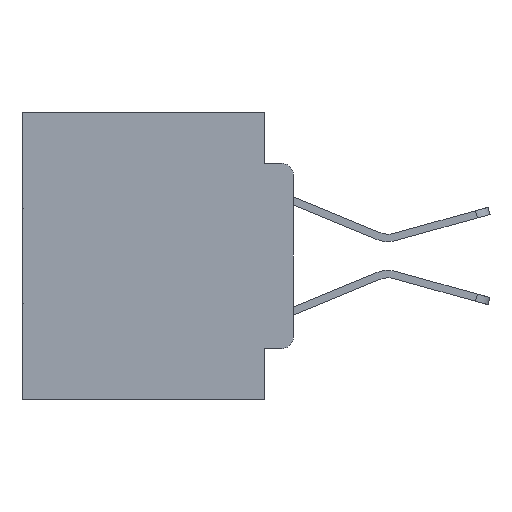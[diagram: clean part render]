
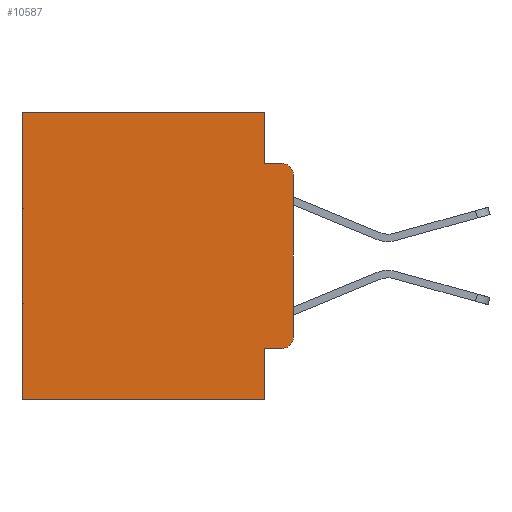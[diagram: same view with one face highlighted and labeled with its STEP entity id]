
A CAD part, left-side view. The second image highlights one B-rep face of the part: STEP entity #10587.
In plain terms, the highlighted planar face has unit normal (-1, 0, 0).
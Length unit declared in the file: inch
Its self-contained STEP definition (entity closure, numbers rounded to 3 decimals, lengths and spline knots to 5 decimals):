
#143 = CARTESIAN_POINT ( 'NONE',  ( 0.298, 0.02, -0.0885 ) ) ;
#873 = DIRECTION ( 'NONE',  ( 0., -1., 0. ) ) ;
#1125 = CARTESIAN_POINT ( 'NONE',  ( 0.298, 0.051, -0.0885 ) ) ;
#1357 = VERTEX_POINT ( 'NONE', #6436 ) ;
#2294 = DIRECTION ( 'NONE',  ( -1., 0., 0. ) ) ;
#2396 = CARTESIAN_POINT ( 'NONE',  ( 0.298, 0.051, -0.4115 ) ) ;
#3027 = AXIS2_PLACEMENT_3D ( 'NONE', #17320, #2294, #19782 ) ;
#3093 = ORIENTED_EDGE ( 'NONE', *, *, #9469, .F. ) ;
#3210 = EDGE_CURVE ( 'NONE', #11670, #21237, #19409, .T. ) ;
#3668 = CARTESIAN_POINT ( 'NONE',  ( 0.298, 0.051, 0. ) ) ;
#4072 = DIRECTION ( 'NONE',  ( -1., 0., 0. ) ) ;
#4357 = CARTESIAN_POINT ( 'NONE',  ( 0.298, 0., 0. ) ) ;
#4598 = ORIENTED_EDGE ( 'NONE', *, *, #27001, .F. ) ;
#5190 = VECTOR ( 'NONE', #873, 39.37008 ) ;
#5524 = EDGE_CURVE ( 'NONE', #11444, #10542, #6011, .T. ) ;
#6011 = LINE ( 'NONE', #9923, #5190 ) ;
#6436 = CARTESIAN_POINT ( 'NONE',  ( 0.298, 0.051, 0. ) ) ;
#6443 = CARTESIAN_POINT ( 'NONE',  ( 0.298, 0.051, -0.4115 ) ) ;
#6484 = VECTOR ( 'NONE', #22529, 39.37008 ) ;
#7074 = VERTEX_POINT ( 'NONE', #31176 ) ;
#7345 = CARTESIAN_POINT ( 'NONE',  ( 0.298, 0.051, 0. ) ) ;
#9018 = AXIS2_PLACEMENT_3D ( 'NONE', #19040, #4072, #21512 ) ;
#9428 = ORIENTED_EDGE ( 'NONE', *, *, #3210, .T. ) ;
#9469 = EDGE_CURVE ( 'NONE', #10667, #11246, #15210, .T. ) ;
#9923 = CARTESIAN_POINT ( 'NONE',  ( 0.298, 0.051, -0.0885 ) ) ;
#10056 = CARTESIAN_POINT ( 'NONE',  ( 0.298, 0.473, 0. ) ) ;
#10485 = ORIENTED_EDGE ( 'NONE', *, *, #21283, .F. ) ;
#10542 = VERTEX_POINT ( 'NONE', #143 ) ;
#10587 = ADVANCED_FACE ( 'NONE', ( #28398 ), #27538, .F. ) ;
#10667 = VERTEX_POINT ( 'NONE', #25426 ) ;
#11131 = DIRECTION ( 'NONE',  ( 0., 0., -1. ) ) ;
#11246 = VERTEX_POINT ( 'NONE', #20359 ) ;
#11261 = ORIENTED_EDGE ( 'NONE', *, *, #27613, .T. ) ;
#11444 = VERTEX_POINT ( 'NONE', #1125 ) ;
#11647 = EDGE_CURVE ( 'NONE', #21237, #11246, #26101, .T. ) ;
#11670 = VERTEX_POINT ( 'NONE', #2396 ) ;
#11968 = DIRECTION ( 'NONE',  ( 0., 1., 0. ) ) ;
#12055 = VECTOR ( 'NONE', #27995, 39.37008 ) ;
#12157 = VECTOR ( 'NONE', #22252, 39.37008 ) ;
#12574 = ORIENTED_EDGE ( 'NONE', *, *, #11647, .T. ) ;
#13023 = DIRECTION ( 'NONE',  ( 1., 0., 0. ) ) ;
#13167 = LINE ( 'NONE', #10056, #6484 ) ;
#13944 = EDGE_CURVE ( 'NONE', #1357, #11444, #25186, .T. ) ;
#14092 = CARTESIAN_POINT ( 'NONE',  ( 0.298, 0., -0.5 ) ) ;
#15188 = LINE ( 'NONE', #3668, #21707 ) ;
#15210 = LINE ( 'NONE', #26027, #28102 ) ;
#16314 = LINE ( 'NONE', #4357, #26168 ) ;
#16788 = DIRECTION ( 'NONE',  ( 0., 1., 0. ) ) ;
#17238 = VERTEX_POINT ( 'NONE', #30618 ) ;
#17320 = CARTESIAN_POINT ( 'NONE',  ( 0.298, 0.02, -0.3915 ) ) ;
#18727 = VERTEX_POINT ( 'NONE', #20818 ) ;
#18994 = EDGE_LOOP ( 'NONE', ( #3093, #11261, #31381, #22961, #22695, #27211, #10485, #4598, #9428, #12574 ) ) ;
#19040 = CARTESIAN_POINT ( 'NONE',  ( 0.298, 0.02, -0.1085 ) ) ;
#19409 = LINE ( 'NONE', #6443, #12055 ) ;
#19615 = EDGE_CURVE ( 'NONE', #1357, #18727, #16314, .T. ) ;
#19782 = DIRECTION ( 'NONE',  ( 0., 0., -1. ) ) ;
#20359 = CARTESIAN_POINT ( 'NONE',  ( 0.298, 0., -0.3915 ) ) ;
#20399 = CARTESIAN_POINT ( 'NONE',  ( 0.298, 0., 0. ) ) ;
#20818 = CARTESIAN_POINT ( 'NONE',  ( 0.298, 0.473, 0. ) ) ;
#21217 = DIRECTION ( 'NONE',  ( 0., 0., -1. ) ) ;
#21237 = VERTEX_POINT ( 'NONE', #30986 ) ;
#21283 = EDGE_CURVE ( 'NONE', #7074, #17238, #27193, .T. ) ;
#21512 = DIRECTION ( 'NONE',  ( 0., 0., -1. ) ) ;
#21707 = VECTOR ( 'NONE', #11131, 39.37008 ) ;
#22187 = EDGE_CURVE ( 'NONE', #18727, #17238, #13167, .T. ) ;
#22252 = DIRECTION ( 'NONE',  ( 0., 0., -1. ) ) ;
#22529 = DIRECTION ( 'NONE',  ( 0., 0., -1. ) ) ;
#22695 = ORIENTED_EDGE ( 'NONE', *, *, #19615, .T. ) ;
#22961 = ORIENTED_EDGE ( 'NONE', *, *, #13944, .F. ) ;
#25186 = LINE ( 'NONE', #7345, #12157 ) ;
#25426 = CARTESIAN_POINT ( 'NONE',  ( 0.298, 0., -0.1085 ) ) ;
#26027 = CARTESIAN_POINT ( 'NONE',  ( 0.298, 0., 0. ) ) ;
#26101 = CIRCLE ( 'NONE', #3027, 0.02 ) ;
#26168 = VECTOR ( 'NONE', #11968, 39.37008 ) ;
#27001 = EDGE_CURVE ( 'NONE', #11670, #7074, #15188, .T. ) ;
#27193 = LINE ( 'NONE', #14092, #31205 ) ;
#27211 = ORIENTED_EDGE ( 'NONE', *, *, #22187, .T. ) ;
#27538 = PLANE ( 'NONE',  #30187 ) ;
#27613 = EDGE_CURVE ( 'NONE', #10667, #10542, #29117, .T. ) ;
#27995 = DIRECTION ( 'NONE',  ( 0., -1., 0. ) ) ;
#28102 = VECTOR ( 'NONE', #21217, 39.37008 ) ;
#28398 = FACE_OUTER_BOUND ( 'NONE', #18994, .T. ) ;
#29117 = CIRCLE ( 'NONE', #9018, 0.02 ) ;
#30006 = DIRECTION ( 'NONE',  ( 0., 0., -1. ) ) ;
#30187 = AXIS2_PLACEMENT_3D ( 'NONE', #20399, #13023, #30006 ) ;
#30618 = CARTESIAN_POINT ( 'NONE',  ( 0.298, 0.473, -0.5 ) ) ;
#30986 = CARTESIAN_POINT ( 'NONE',  ( 0.298, 0.02, -0.4115 ) ) ;
#31176 = CARTESIAN_POINT ( 'NONE',  ( 0.298, 0.051, -0.5 ) ) ;
#31205 = VECTOR ( 'NONE', #16788, 39.37008 ) ;
#31381 = ORIENTED_EDGE ( 'NONE', *, *, #5524, .F. ) ;
